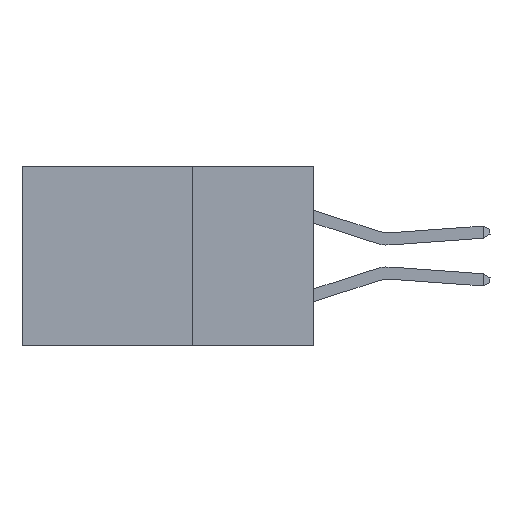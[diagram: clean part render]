
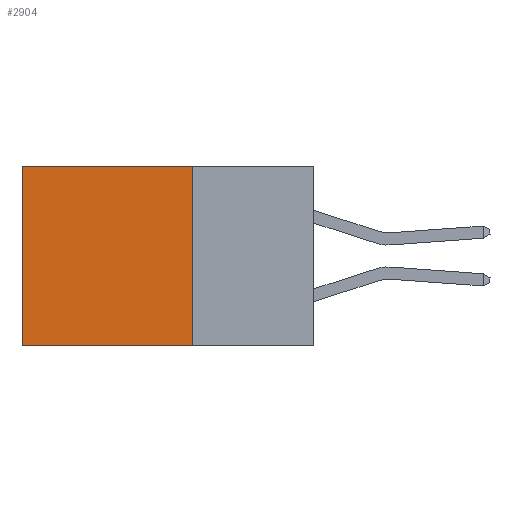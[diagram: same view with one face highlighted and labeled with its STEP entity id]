
A CAD part, left-side view. The second image highlights one B-rep face of the part: STEP entity #2904.
In plain terms, the highlighted planar face has unit normal (-1, 0, 0).
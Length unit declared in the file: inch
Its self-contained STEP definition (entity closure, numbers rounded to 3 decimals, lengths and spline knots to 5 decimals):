
#757 = ORIENTED_EDGE ( 'NONE', *, *, #4460, .F. ) ;
#1005 = CARTESIAN_POINT ( 'NONE',  ( 0.2875, 0.6, -0.37 ) ) ;
#1274 = PLANE ( 'NONE',  #4678 ) ;
#1593 = CARTESIAN_POINT ( 'NONE',  ( 0.2875, 0.25, -0.37 ) ) ;
#1696 = VERTEX_POINT ( 'NONE', #18487 ) ;
#2904 = ADVANCED_FACE ( 'NONE', ( #21764 ), #1274, .F. ) ;
#3509 = DIRECTION ( 'NONE',  ( 0., 0., -1. ) ) ;
#4457 = CARTESIAN_POINT ( 'NONE',  ( 0.2875, 0.6, 0. ) ) ;
#4460 = EDGE_CURVE ( 'NONE', #1696, #12328, #18454, .T. ) ;
#4678 = AXIS2_PLACEMENT_3D ( 'NONE', #21898, #18285, #20009 ) ;
#5100 = DIRECTION ( 'NONE',  ( 0., 1., 0. ) ) ;
#5763 = VECTOR ( 'NONE', #6717, 39.37008 ) ;
#6263 = VECTOR ( 'NONE', #15196, 39.37008 ) ;
#6717 = DIRECTION ( 'NONE',  ( 0., 1., 0. ) ) ;
#8863 = CARTESIAN_POINT ( 'NONE',  ( 0.2875, 0.25, 0. ) ) ;
#11802 = VERTEX_POINT ( 'NONE', #4457 ) ;
#12112 = LINE ( 'NONE', #8863, #21644 ) ;
#12277 = ORIENTED_EDGE ( 'NONE', *, *, #13970, .F. ) ;
#12328 = VERTEX_POINT ( 'NONE', #1005 ) ;
#12344 = CARTESIAN_POINT ( 'NONE',  ( 0.2875, 0.25, 0. ) ) ;
#12559 = ORIENTED_EDGE ( 'NONE', *, *, #16289, .T. ) ;
#13970 = EDGE_CURVE ( 'NONE', #19991, #1696, #12112, .T. ) ;
#14494 = EDGE_CURVE ( 'NONE', #11802, #12328, #21357, .T. ) ;
#14549 = VECTOR ( 'NONE', #5100, 39.37008 ) ;
#15196 = DIRECTION ( 'NONE',  ( 0., 0., -1. ) ) ;
#16289 = EDGE_CURVE ( 'NONE', #19991, #11802, #20596, .T. ) ;
#18285 = DIRECTION ( 'NONE',  ( 1., 0., 0. ) ) ;
#18454 = LINE ( 'NONE', #1593, #14549 ) ;
#18487 = CARTESIAN_POINT ( 'NONE',  ( 0.2875, 0.25, -0.37 ) ) ;
#19929 = ORIENTED_EDGE ( 'NONE', *, *, #14494, .T. ) ;
#19991 = VERTEX_POINT ( 'NONE', #24103 ) ;
#20009 = DIRECTION ( 'NONE',  ( 0., 0., -1. ) ) ;
#20596 = LINE ( 'NONE', #12344, #5763 ) ;
#20852 = CARTESIAN_POINT ( 'NONE',  ( 0.2875, 0.6, 0. ) ) ;
#21357 = LINE ( 'NONE', #20852, #6263 ) ;
#21644 = VECTOR ( 'NONE', #3509, 39.37008 ) ;
#21764 = FACE_OUTER_BOUND ( 'NONE', #23738, .T. ) ;
#21898 = CARTESIAN_POINT ( 'NONE',  ( 0.2875, 0.25, 0. ) ) ;
#23738 = EDGE_LOOP ( 'NONE', ( #19929, #757, #12277, #12559 ) ) ;
#24103 = CARTESIAN_POINT ( 'NONE',  ( 0.2875, 0.25, 0. ) ) ;
